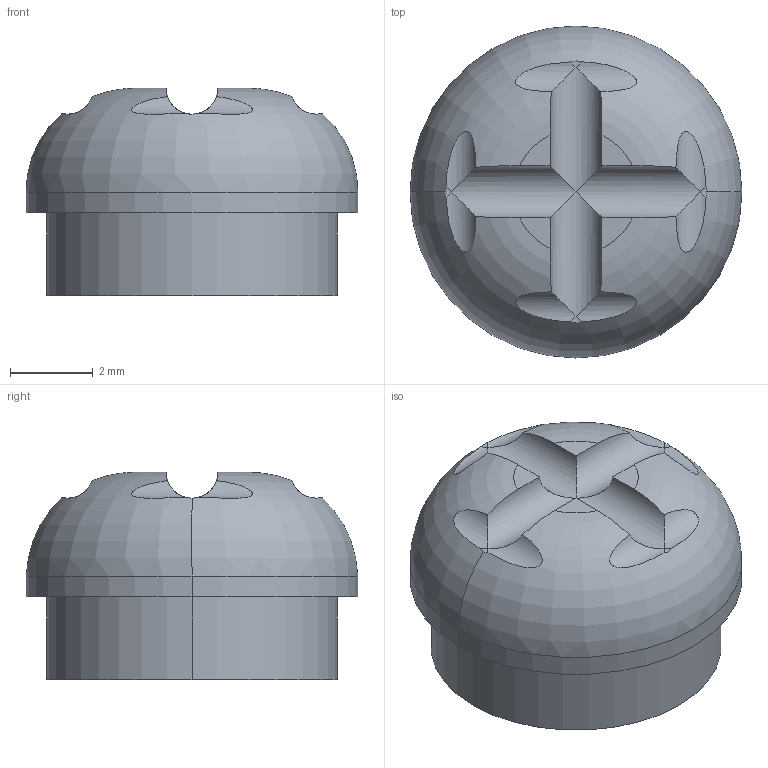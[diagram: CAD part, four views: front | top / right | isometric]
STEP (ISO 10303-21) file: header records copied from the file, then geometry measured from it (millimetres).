
FILE_DESCRIPTION (( 'STEP AP214' ), '1' );
FILE_NAME ('Frame_Pins_Cap.STEP', '2014-02-20T01:50:31', ( '' ), ( '' ), 'SwSTEP 2.0', 'SolidWorks 2013', '' );
FILE_SCHEMA (( 'AUTOMOTIVE_DESIGN' ));
Length unit declared in the file: millimetre
Products named in the file (1): Frame_Pins_Cap
Bounding box: 8 x 8 x 5 mm (x, y, z)
Volume: 153.5 mm3; surface area: 226.1 mm2
Topology: 1 solids, 1 shells, 31 faces, 74 edges, 47 vertices
Faces by surface type: cylinder 22, plane 7, torus 2
Entity records: 1110 total; most frequent: CARTESIAN_POINT 443, ORIENTED_EDGE 148, DIRECTION 114, EDGE_CURVE 74, AXIS2_PLACEMENT_3D 50, VERTEX_POINT 47, EDGE_LOOP 33, ADVANCED_FACE 31
